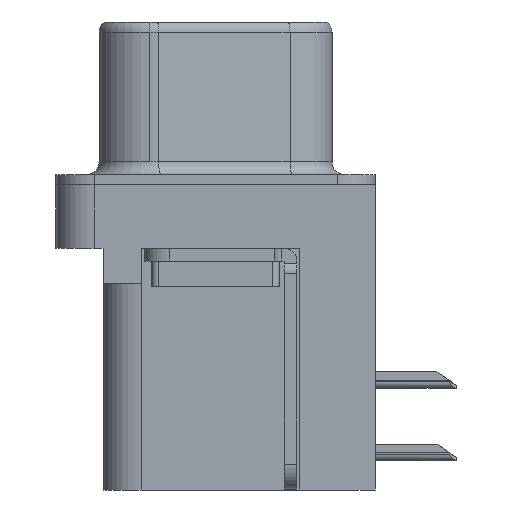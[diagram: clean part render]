
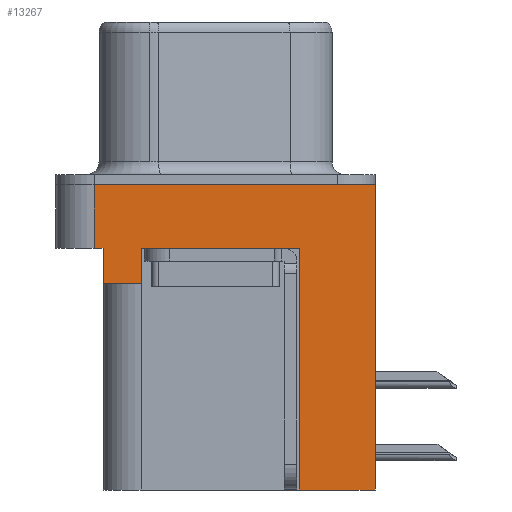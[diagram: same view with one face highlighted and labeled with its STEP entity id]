
A CAD part, left-side view. The second image highlights one B-rep face of the part: STEP entity #13267.
In plain terms, the highlighted planar face has unit normal (-1, 0, 0).
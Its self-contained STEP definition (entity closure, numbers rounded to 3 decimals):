
#68 = CARTESIAN_POINT ( 'NONE',  ( -2.91, -6.275, -2.5 ) ) ;
#245 = CARTESIAN_POINT ( 'NONE',  ( -2.91, -6.275, 0. ) ) ;
#1087 = VECTOR ( 'NONE', #12241, 1000. ) ;
#1093 = ORIENTED_EDGE ( 'NONE', *, *, #6878, .F. ) ;
#1509 = VECTOR ( 'NONE', #16342, 1000. ) ;
#1623 = EDGE_CURVE ( 'NONE', #1699, #15395, #22411, .T. ) ;
#1699 = VERTEX_POINT ( 'NONE', #18652 ) ;
#3496 = VERTEX_POINT ( 'NONE', #6244 ) ;
#3589 = CARTESIAN_POINT ( 'NONE',  ( -2.91, -6.275, -2.5 ) ) ;
#4725 = VECTOR ( 'NONE', #16024, 1000. ) ;
#4800 = DIRECTION ( 'NONE',  ( 0., 0., 1. ) ) ;
#5475 = ORIENTED_EDGE ( 'NONE', *, *, #20073, .F. ) ;
#5571 = FACE_OUTER_BOUND ( 'NONE', #15337, .T. ) ;
#5605 = DIRECTION ( 'NONE',  ( 0., 1., 0. ) ) ;
#6090 = CARTESIAN_POINT ( 'NONE',  ( -2.91, 4.425, -3.9 ) ) ;
#6244 = CARTESIAN_POINT ( 'NONE',  ( -2.91, 2.895, -2.5 ) ) ;
#6295 = DIRECTION ( 'NONE',  ( 0., 0., 1. ) ) ;
#6878 = EDGE_CURVE ( 'NONE', #20044, #7970, #16806, .T. ) ;
#7073 = LINE ( 'NONE', #9974, #1509 ) ;
#7970 = VERTEX_POINT ( 'NONE', #6090 ) ;
#8122 = VERTEX_POINT ( 'NONE', #245 ) ;
#8233 = DIRECTION ( 'NONE',  ( -1., 0., 0. ) ) ;
#8320 = CARTESIAN_POINT ( 'NONE',  ( -2.91, -6.275, -2.5 ) ) ;
#8899 = CARTESIAN_POINT ( 'NONE',  ( -2.91, 2.895, -3.9 ) ) ;
#9106 = ORIENTED_EDGE ( 'NONE', *, *, #11551, .T. ) ;
#9478 = ORIENTED_EDGE ( 'NONE', *, *, #13997, .F. ) ;
#9699 = EDGE_CURVE ( 'NONE', #1699, #18921, #7073, .T. ) ;
#9796 = CARTESIAN_POINT ( 'NONE',  ( -2.91, 2.895, -3.9 ) ) ;
#9974 = CARTESIAN_POINT ( 'NONE',  ( -2.91, 4.775, -2.5 ) ) ;
#10133 = ORIENTED_EDGE ( 'NONE', *, *, #16604, .T. ) ;
#10215 = VECTOR ( 'NONE', #4800, 1000. ) ;
#10553 = LINE ( 'NONE', #14439, #15036 ) ;
#10714 = VECTOR ( 'NONE', #24337, 1000. ) ;
#10745 = AXIS2_PLACEMENT_3D ( 'NONE', #8320, #8233, #6295 ) ;
#10752 = DIRECTION ( 'NONE',  ( 0., -1., 0. ) ) ;
#11430 = ORIENTED_EDGE ( 'NONE', *, *, #14624, .F. ) ;
#11551 = EDGE_CURVE ( 'NONE', #13929, #8122, #20457, .T. ) ;
#11775 = VECTOR ( 'NONE', #14945, 1000. ) ;
#12241 = DIRECTION ( 'NONE',  ( 0., 0., 1. ) ) ;
#12293 = CARTESIAN_POINT ( 'NONE',  ( -2.91, -6.275, -12. ) ) ;
#12628 = DIRECTION ( 'NONE',  ( 0., 0., 1. ) ) ;
#12950 = VERTEX_POINT ( 'NONE', #15185 ) ;
#13267 = ADVANCED_FACE ( 'NONE', ( #5571 ), #16148, .T. ) ;
#13500 = ORIENTED_EDGE ( 'NONE', *, *, #19500, .F. ) ;
#13929 = VERTEX_POINT ( 'NONE', #12293 ) ;
#13997 = EDGE_CURVE ( 'NONE', #7970, #15395, #10553, .T. ) ;
#14338 = VECTOR ( 'NONE', #18212, 1000. ) ;
#14439 = CARTESIAN_POINT ( 'NONE',  ( -2.91, 4.425, -3.9 ) ) ;
#14624 = EDGE_CURVE ( 'NONE', #13929, #12950, #23235, .T. ) ;
#14945 = DIRECTION ( 'NONE',  ( 0., -1., 0. ) ) ;
#15035 = CARTESIAN_POINT ( 'NONE',  ( -2.91, -6.275, 0. ) ) ;
#15036 = VECTOR ( 'NONE', #12628, 1000. ) ;
#15185 = CARTESIAN_POINT ( 'NONE',  ( -2.91, -3.295, -12. ) ) ;
#15321 = ORIENTED_EDGE ( 'NONE', *, *, #9699, .F. ) ;
#15337 = EDGE_LOOP ( 'NONE', ( #13500, #15321, #24886, #9478, #1093, #10133, #19113, #5475, #11430, #9106 ) ) ;
#15395 = VERTEX_POINT ( 'NONE', #20416 ) ;
#16024 = DIRECTION ( 'NONE',  ( 0., -1., 0. ) ) ;
#16079 = CARTESIAN_POINT ( 'NONE',  ( -2.91, -3.295, -12. ) ) ;
#16148 = PLANE ( 'NONE',  #10745 ) ;
#16161 = CARTESIAN_POINT ( 'NONE',  ( -2.91, -3.295, -12. ) ) ;
#16300 = LINE ( 'NONE', #8899, #10215 ) ;
#16342 = DIRECTION ( 'NONE',  ( 0., 0., 1. ) ) ;
#16604 = EDGE_CURVE ( 'NONE', #20044, #3496, #16300, .T. ) ;
#16806 = LINE ( 'NONE', #18089, #10714 ) ;
#17033 = LINE ( 'NONE', #18729, #22525 ) ;
#18089 = CARTESIAN_POINT ( 'NONE',  ( -2.91, 4.425, -3.9 ) ) ;
#18212 = DIRECTION ( 'NONE',  ( 0., 0., 1. ) ) ;
#18652 = CARTESIAN_POINT ( 'NONE',  ( -2.91, 4.775, -2.5 ) ) ;
#18729 = CARTESIAN_POINT ( 'NONE',  ( -2.91, -6.275, -2.5 ) ) ;
#18921 = VERTEX_POINT ( 'NONE', #19045 ) ;
#19045 = CARTESIAN_POINT ( 'NONE',  ( -2.91, 4.775, 0. ) ) ;
#19113 = ORIENTED_EDGE ( 'NONE', *, *, #24635, .T. ) ;
#19499 = LINE ( 'NONE', #15035, #11775 ) ;
#19500 = EDGE_CURVE ( 'NONE', #18921, #8122, #19499, .T. ) ;
#20044 = VERTEX_POINT ( 'NONE', #9796 ) ;
#20073 = EDGE_CURVE ( 'NONE', #12950, #21791, #21410, .T. ) ;
#20416 = CARTESIAN_POINT ( 'NONE',  ( -2.91, 4.425, -2.5 ) ) ;
#20457 = LINE ( 'NONE', #68, #1087 ) ;
#21410 = LINE ( 'NONE', #16161, #14338 ) ;
#21791 = VERTEX_POINT ( 'NONE', #23942 ) ;
#22411 = LINE ( 'NONE', #3589, #4725 ) ;
#22525 = VECTOR ( 'NONE', #10752, 1000. ) ;
#22904 = VECTOR ( 'NONE', #5605, 1000. ) ;
#23235 = LINE ( 'NONE', #16079, #22904 ) ;
#23942 = CARTESIAN_POINT ( 'NONE',  ( -2.91, -3.295, -2.5 ) ) ;
#24337 = DIRECTION ( 'NONE',  ( 0., 1., 0. ) ) ;
#24635 = EDGE_CURVE ( 'NONE', #3496, #21791, #17033, .T. ) ;
#24886 = ORIENTED_EDGE ( 'NONE', *, *, #1623, .T. ) ;
